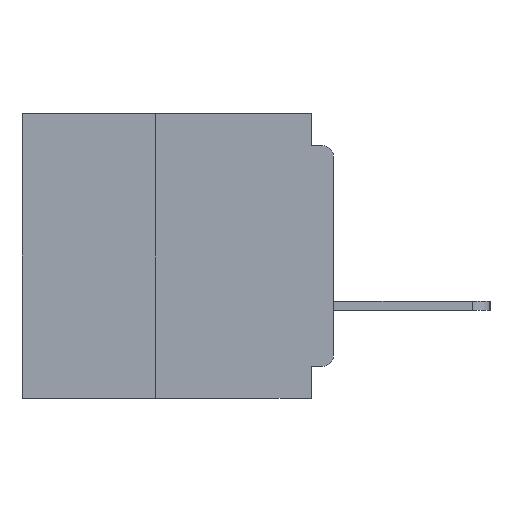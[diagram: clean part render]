
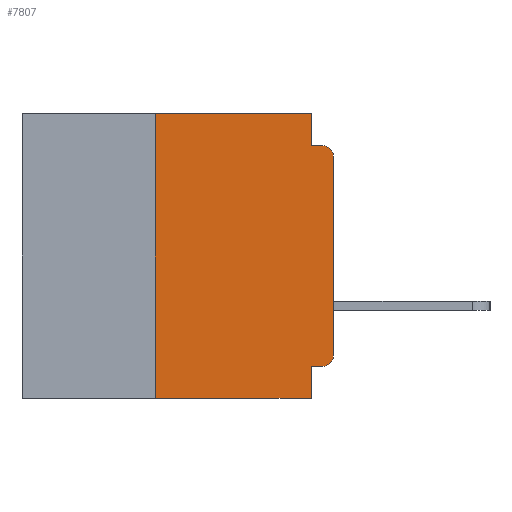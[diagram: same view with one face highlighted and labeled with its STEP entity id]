
A CAD part, left-side view. The second image highlights one B-rep face of the part: STEP entity #7807.
In plain terms, the highlighted planar face has unit normal (-1, 0, 0).
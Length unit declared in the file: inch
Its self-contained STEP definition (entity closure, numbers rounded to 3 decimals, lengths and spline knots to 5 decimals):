
#201 = VERTEX_POINT ( 'NONE', #7073 ) ;
#597 = VECTOR ( 'NONE', #7326, 39.37008 ) ;
#676 = VECTOR ( 'NONE', #10093, 39.37008 ) ;
#1363 = PLANE ( 'NONE',  #25236 ) ;
#1616 = CARTESIAN_POINT ( 'NONE',  ( 0., 0.031, -0.355 ) ) ;
#2083 = VERTEX_POINT ( 'NONE', #33931 ) ;
#3133 = CARTESIAN_POINT ( 'NONE',  ( 0., 0., -0.045 ) ) ;
#3550 = EDGE_CURVE ( 'NONE', #14851, #11025, #16252, .T. ) ;
#3860 = DIRECTION ( 'NONE',  ( 1., 0., 0. ) ) ;
#4285 = DIRECTION ( 'NONE',  ( 0., 0., -1. ) ) ;
#5062 = ORIENTED_EDGE ( 'NONE', *, *, #15318, .T. ) ;
#5937 = LINE ( 'NONE', #20620, #31152 ) ;
#7070 = CARTESIAN_POINT ( 'NONE',  ( 0., 0.437, 0. ) ) ;
#7073 = CARTESIAN_POINT ( 'NONE',  ( 0., 0.25, 0. ) ) ;
#7326 = DIRECTION ( 'NONE',  ( 0., -1., 0. ) ) ;
#7373 = LINE ( 'NONE', #11554, #20939 ) ;
#7807 = ADVANCED_FACE ( 'NONE', ( #30596 ), #1363, .F. ) ;
#8213 = CARTESIAN_POINT ( 'NONE',  ( 0., 0., -0.06 ) ) ;
#9321 = CARTESIAN_POINT ( 'NONE',  ( 0., 0., -0.355 ) ) ;
#9679 = ORIENTED_EDGE ( 'NONE', *, *, #11629, .F. ) ;
#9709 = VERTEX_POINT ( 'NONE', #26241 ) ;
#10093 = DIRECTION ( 'NONE',  ( 0., 0., 1. ) ) ;
#10964 = ORIENTED_EDGE ( 'NONE', *, *, #31303, .T. ) ;
#11025 = VERTEX_POINT ( 'NONE', #29487 ) ;
#11399 = DIRECTION ( 'NONE',  ( 0., -1., 0. ) ) ;
#11554 = CARTESIAN_POINT ( 'NONE',  ( 0., 0.031, 0. ) ) ;
#11622 = ORIENTED_EDGE ( 'NONE', *, *, #21864, .F. ) ;
#11629 = EDGE_CURVE ( 'NONE', #201, #2083, #15098, .T. ) ;
#12380 = CARTESIAN_POINT ( 'NONE',  ( 0., 0.031, -0.045 ) ) ;
#12411 = CARTESIAN_POINT ( 'NONE',  ( 0., 0.015, -0.34 ) ) ;
#13592 = VECTOR ( 'NONE', #17494, 39.37008 ) ;
#13648 = ORIENTED_EDGE ( 'NONE', *, *, #22178, .T. ) ;
#13686 = EDGE_LOOP ( 'NONE', ( #10964, #13648, #32869, #15482, #9679, #25711, #15985, #23845, #11622, #5062 ) ) ;
#14432 = LINE ( 'NONE', #9321, #13592 ) ;
#14851 = VERTEX_POINT ( 'NONE', #1616 ) ;
#15098 = LINE ( 'NONE', #26206, #597 ) ;
#15104 = DIRECTION ( 'NONE',  ( 0., 0., -1. ) ) ;
#15190 = LINE ( 'NONE', #31625, #676 ) ;
#15248 = EDGE_CURVE ( 'NONE', #2083, #22543, #7373, .T. ) ;
#15318 = EDGE_CURVE ( 'NONE', #28318, #30812, #33341, .T. ) ;
#15482 = ORIENTED_EDGE ( 'NONE', *, *, #15248, .F. ) ;
#15650 = VERTEX_POINT ( 'NONE', #8213 ) ;
#15985 = ORIENTED_EDGE ( 'NONE', *, *, #25977, .T. ) ;
#16172 = CARTESIAN_POINT ( 'NONE',  ( 0., 0.015, -0.06 ) ) ;
#16252 = LINE ( 'NONE', #19827, #29631 ) ;
#16997 = DIRECTION ( 'NONE',  ( 0., 0., -1. ) ) ;
#17017 = VECTOR ( 'NONE', #11399, 39.37008 ) ;
#17274 = DIRECTION ( 'NONE',  ( 0., -1., 0. ) ) ;
#17494 = DIRECTION ( 'NONE',  ( 0., 1., 0. ) ) ;
#18832 = VECTOR ( 'NONE', #17274, 39.37008 ) ;
#18906 = DIRECTION ( 'NONE',  ( 0., 0., -1. ) ) ;
#19408 = EDGE_CURVE ( 'NONE', #23852, #201, #15190, .T. ) ;
#19719 = DIRECTION ( 'NONE',  ( 0., 0., -1. ) ) ;
#19827 = CARTESIAN_POINT ( 'NONE',  ( 0., 0.031, -0.4 ) ) ;
#20620 = CARTESIAN_POINT ( 'NONE',  ( 0., 0., 0. ) ) ;
#20939 = VECTOR ( 'NONE', #16997, 39.37008 ) ;
#21288 = AXIS2_PLACEMENT_3D ( 'NONE', #16172, #34746, #18906 ) ;
#21864 = EDGE_CURVE ( 'NONE', #28318, #14851, #14432, .T. ) ;
#22178 = EDGE_CURVE ( 'NONE', #15650, #9709, #24940, .T. ) ;
#22543 = VERTEX_POINT ( 'NONE', #12380 ) ;
#23331 = DIRECTION ( 'NONE',  ( 0., 0., 1. ) ) ;
#23845 = ORIENTED_EDGE ( 'NONE', *, *, #3550, .F. ) ;
#23852 = VERTEX_POINT ( 'NONE', #34585 ) ;
#24940 = CIRCLE ( 'NONE', #21288, 0.015 ) ;
#25236 = AXIS2_PLACEMENT_3D ( 'NONE', #7070, #3860, #4285 ) ;
#25711 = ORIENTED_EDGE ( 'NONE', *, *, #19408, .F. ) ;
#25953 = LINE ( 'NONE', #33198, #18832 ) ;
#25977 = EDGE_CURVE ( 'NONE', #23852, #11025, #25953, .T. ) ;
#26206 = CARTESIAN_POINT ( 'NONE',  ( 0., 0.437, 0. ) ) ;
#26241 = CARTESIAN_POINT ( 'NONE',  ( 0., 0.015, -0.045 ) ) ;
#28318 = VERTEX_POINT ( 'NONE', #31677 ) ;
#29487 = CARTESIAN_POINT ( 'NONE',  ( 0., 0.031, -0.4 ) ) ;
#29631 = VECTOR ( 'NONE', #19719, 39.37008 ) ;
#30596 = FACE_OUTER_BOUND ( 'NONE', #13686, .T. ) ;
#30812 = VERTEX_POINT ( 'NONE', #34842 ) ;
#30900 = EDGE_CURVE ( 'NONE', #22543, #9709, #31991, .T. ) ;
#31094 = DIRECTION ( 'NONE',  ( -1., 0., 0. ) ) ;
#31152 = VECTOR ( 'NONE', #23331, 39.37008 ) ;
#31303 = EDGE_CURVE ( 'NONE', #30812, #15650, #5937, .T. ) ;
#31625 = CARTESIAN_POINT ( 'NONE',  ( 0., 0.25, -0.4 ) ) ;
#31677 = CARTESIAN_POINT ( 'NONE',  ( 0., 0.015, -0.355 ) ) ;
#31991 = LINE ( 'NONE', #3133, #17017 ) ;
#32869 = ORIENTED_EDGE ( 'NONE', *, *, #30900, .F. ) ;
#33198 = CARTESIAN_POINT ( 'NONE',  ( 0., 0.437, -0.4 ) ) ;
#33341 = CIRCLE ( 'NONE', #34614, 0.015 ) ;
#33931 = CARTESIAN_POINT ( 'NONE',  ( 0., 0.031, 0. ) ) ;
#34585 = CARTESIAN_POINT ( 'NONE',  ( 0., 0.25, -0.4 ) ) ;
#34614 = AXIS2_PLACEMENT_3D ( 'NONE', #12411, #31094, #15104 ) ;
#34746 = DIRECTION ( 'NONE',  ( -1., 0., 0. ) ) ;
#34842 = CARTESIAN_POINT ( 'NONE',  ( 0., 0., -0.34 ) ) ;
